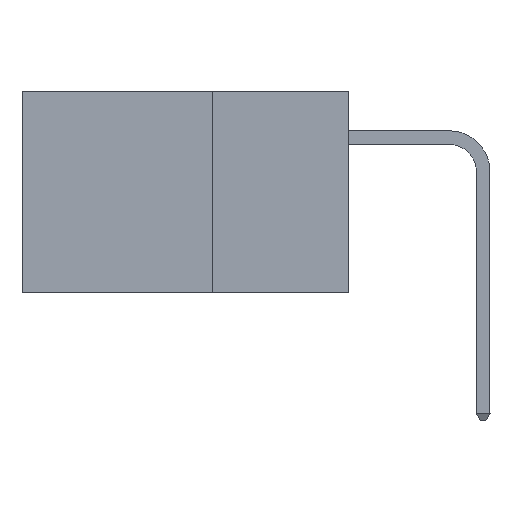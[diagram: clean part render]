
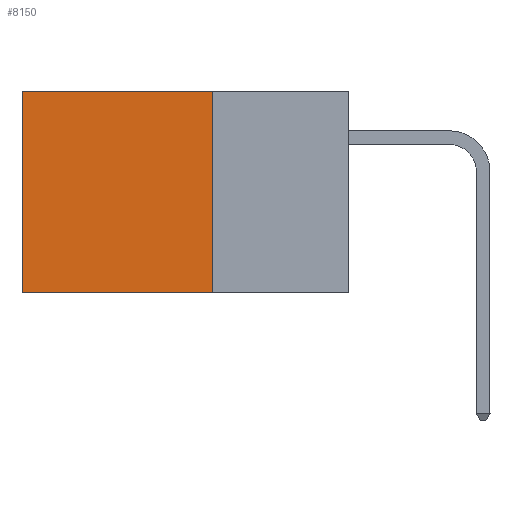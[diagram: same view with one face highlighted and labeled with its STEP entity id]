
A CAD part, left-side view. The second image highlights one B-rep face of the part: STEP entity #8150.
In plain terms, the highlighted planar face has unit normal (-1, 0, 0).
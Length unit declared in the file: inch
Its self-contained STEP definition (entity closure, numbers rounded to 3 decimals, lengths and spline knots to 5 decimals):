
#289 = EDGE_CURVE ( 'NONE', #9899, #10766, #582, .T. ) ;
#499 = ORIENTED_EDGE ( 'NONE', *, *, #289, .F. ) ;
#582 = LINE ( 'NONE', #9496, #10604 ) ;
#588 = ORIENTED_EDGE ( 'NONE', *, *, #16847, .T. ) ;
#965 = CARTESIAN_POINT ( 'NONE',  ( 0.2875, 0.6, 0. ) ) ;
#1297 = DIRECTION ( 'NONE',  ( 0., 0., -1. ) ) ;
#2299 = CARTESIAN_POINT ( 'NONE',  ( 0.2875, 0.25, 0. ) ) ;
#2543 = LINE ( 'NONE', #15154, #15064 ) ;
#3599 = EDGE_CURVE ( 'NONE', #10766, #10213, #7928, .T. ) ;
#3857 = AXIS2_PLACEMENT_3D ( 'NONE', #2299, #5792, #12828 ) ;
#3875 = CARTESIAN_POINT ( 'NONE',  ( 0.2875, 0.6, 0. ) ) ;
#4451 = DIRECTION ( 'NONE',  ( 0., 1., 0. ) ) ;
#5460 = ORIENTED_EDGE ( 'NONE', *, *, #3599, .F. ) ;
#5474 = ORIENTED_EDGE ( 'NONE', *, *, #15475, .T. ) ;
#5792 = DIRECTION ( 'NONE',  ( 1., 0., 0. ) ) ;
#7928 = LINE ( 'NONE', #16714, #16735 ) ;
#8150 = ADVANCED_FACE ( 'NONE', ( #14567 ), #21620, .F. ) ;
#8351 = VERTEX_POINT ( 'NONE', #3875 ) ;
#9244 = CARTESIAN_POINT ( 'NONE',  ( 0.2875, 0.6, -0.37 ) ) ;
#9496 = CARTESIAN_POINT ( 'NONE',  ( 0.2875, 0.25, 0. ) ) ;
#9506 = DIRECTION ( 'NONE',  ( 0., 1., 0. ) ) ;
#9899 = VERTEX_POINT ( 'NONE', #17729 ) ;
#10213 = VERTEX_POINT ( 'NONE', #9244 ) ;
#10604 = VECTOR ( 'NONE', #10990, 39.37008 ) ;
#10766 = VERTEX_POINT ( 'NONE', #13350 ) ;
#10990 = DIRECTION ( 'NONE',  ( 0., 0., -1. ) ) ;
#12828 = DIRECTION ( 'NONE',  ( 0., 0., -1. ) ) ;
#12988 = LINE ( 'NONE', #965, #17996 ) ;
#13350 = CARTESIAN_POINT ( 'NONE',  ( 0.2875, 0.25, -0.37 ) ) ;
#14567 = FACE_OUTER_BOUND ( 'NONE', #18757, .T. ) ;
#15064 = VECTOR ( 'NONE', #9506, 39.37008 ) ;
#15154 = CARTESIAN_POINT ( 'NONE',  ( 0.2875, 0.25, 0. ) ) ;
#15475 = EDGE_CURVE ( 'NONE', #9899, #8351, #2543, .T. ) ;
#16714 = CARTESIAN_POINT ( 'NONE',  ( 0.2875, 0.25, -0.37 ) ) ;
#16735 = VECTOR ( 'NONE', #4451, 39.37008 ) ;
#16847 = EDGE_CURVE ( 'NONE', #8351, #10213, #12988, .T. ) ;
#17729 = CARTESIAN_POINT ( 'NONE',  ( 0.2875, 0.25, 0. ) ) ;
#17996 = VECTOR ( 'NONE', #1297, 39.37008 ) ;
#18757 = EDGE_LOOP ( 'NONE', ( #588, #5460, #499, #5474 ) ) ;
#21620 = PLANE ( 'NONE',  #3857 ) ;
